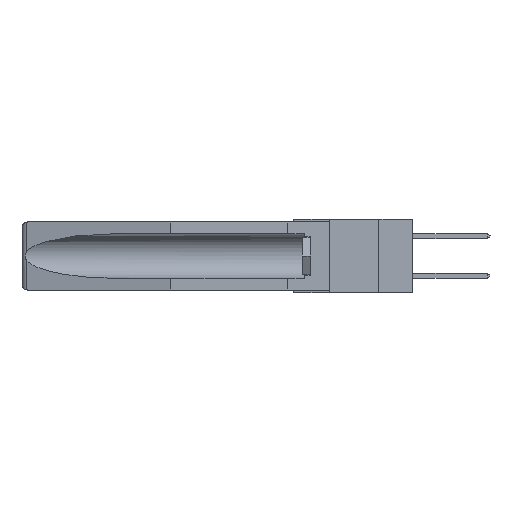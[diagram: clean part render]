
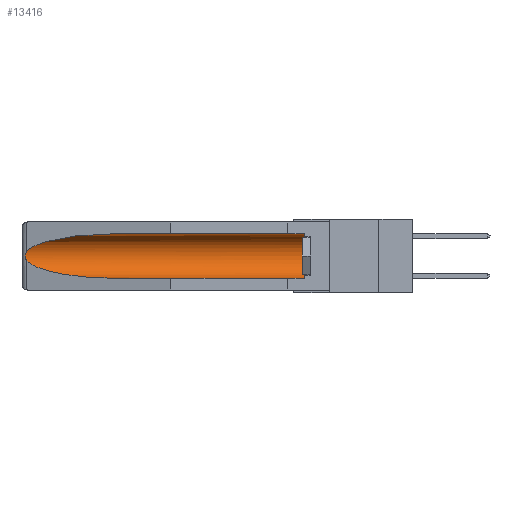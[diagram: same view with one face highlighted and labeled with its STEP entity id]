
A CAD part, left-side view. The second image highlights one B-rep face of the part: STEP entity #13416.
In plain terms, the highlighted cylindrical face has radius 2.857 mm (diameter 5.715 mm), a partial arc.
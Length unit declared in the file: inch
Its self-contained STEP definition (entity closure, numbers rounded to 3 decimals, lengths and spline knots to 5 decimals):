
#268 = CARTESIAN_POINT ( 'NONE',  ( 0.21114, 1.30732, -0.284 ) ) ;
#536 = DIRECTION ( 'NONE',  ( 0., 0., 1. ) ) ;
#1988 = LINE ( 'NONE', #3921, #26443 ) ;
#2520 = CARTESIAN_POINT ( 'NONE',  ( 0.2675, 1.53308, -0.17534 ) ) ;
#2658 = FACE_OUTER_BOUND ( 'NONE', #21291, .T. ) ;
#3213 = ORIENTED_EDGE ( 'NONE', *, *, #4659, .T. ) ;
#3408 = CYLINDRICAL_SURFACE ( 'NONE', #22263, 0.1125 ) ;
#3654 = EDGE_CURVE ( 'NONE', #27541, #6401, #23928, .T. ) ;
#3921 = CARTESIAN_POINT ( 'NONE',  ( 0.155, -0.30754, -0.059 ) ) ;
#4659 = EDGE_CURVE ( 'NONE', #10748, #25160, #1988, .T. ) ;
#5282 = CARTESIAN_POINT ( 'NONE',  ( 0.26537, 1.52718, -0.14972 ) ) ;
#6401 = VERTEX_POINT ( 'NONE', #11095 ) ;
#6407 = CARTESIAN_POINT ( 'NONE',  ( 0.155, 1.07973, -0.059 ) ) ;
#6480 = VECTOR ( 'NONE', #16291, 39.37008 ) ;
#7363 = CARTESIAN_POINT ( 'NONE',  ( 0.26597, 1.52961, -0.15275 ) ) ;
#7473 = CARTESIAN_POINT ( 'NONE',  ( 0.2673, 1.5327, -0.16383 ) ) ;
#7958 = CARTESIAN_POINT ( 'NONE',  ( 0.26537, 1.52718, -0.19328 ) ) ;
#8091 = ORIENTED_EDGE ( 'NONE', *, *, #16795, .T. ) ;
#9112 = CARTESIAN_POINT ( 'NONE',  ( 0.155, 0.126, -0.284 ) ) ;
#9590 = CIRCLE ( 'NONE', #29709, 0.1125 ) ;
#9718 = CARTESIAN_POINT ( 'NONE',  ( 0.26597, 1.5296, -0.19026 ) ) ;
#10748 = VERTEX_POINT ( 'NONE', #13776 ) ;
#11095 = CARTESIAN_POINT ( 'NONE',  ( 0.155, 1.07973, -0.284 ) ) ;
#11285 = EDGE_CURVE ( 'NONE', #25160, #21523, #18745, .T. ) ;
#11732 = CARTESIAN_POINT ( 'NONE',  ( 0.25451, 1.48313, -0.24835 ) ) ;
#12219 = CARTESIAN_POINT ( 'NONE',  ( 0.155, 1.07973, -0.059 ) ) ;
#12221 = CARTESIAN_POINT ( 'NONE',  ( 0.26654, 1.53092, -0.15636 ) ) ;
#13416 = ADVANCED_FACE ( 'NONE', ( #2658 ), #3408, .F. ) ;
#13776 = CARTESIAN_POINT ( 'NONE',  ( 0.155, 0.126, -0.059 ) ) ;
#13847 = CARTESIAN_POINT ( 'NONE',  ( 0.26537, 1.52718, -0.14972 ) ) ;
#15206 = ORIENTED_EDGE ( 'NONE', *, *, #3654, .F. ) ;
#16058 =( BOUNDED_CURVE ( )  B_SPLINE_CURVE ( 3, ( #28630, #11732, #268, #21120 ),
 .UNSPECIFIED., .F., .F. ) 
 B_SPLINE_CURVE_WITH_KNOTS ( ( 4, 4 ),
 ( 0.1948, 1.5708 ),
 .UNSPECIFIED. ) 
 CURVE ( )  GEOMETRIC_REPRESENTATION_ITEM ( )  RATIONAL_B_SPLINE_CURVE ( ( 1., 0.848, 0.848, 1. ) ) 
 REPRESENTATION_ITEM ( '' )  );
#16282 = CARTESIAN_POINT ( 'NONE',  ( 0.25451, 1.48313, -0.09465 ) ) ;
#16291 = DIRECTION ( 'NONE',  ( 0., 1., 0. ) ) ;
#16485 = ORIENTED_EDGE ( 'NONE', *, *, #28296, .T. ) ;
#16735 = CARTESIAN_POINT ( 'NONE',  ( 0.26537, 1.52718, -0.14972 ) ) ;
#16795 = EDGE_CURVE ( 'NONE', #21523, #22930, #18353, .T. ) ;
#17020 = CARTESIAN_POINT ( 'NONE',  ( 0.155, -0.30754, -0.1715 ) ) ;
#17056 = CARTESIAN_POINT ( 'NONE',  ( 0.26537, 1.52718, -0.19328 ) ) ;
#18353 = B_SPLINE_CURVE_WITH_KNOTS ( 'NONE', 3,
 ( #16735, #7363, #12221, #7473, #23977, #2520, #21411, #26237, #9718, #17056 ),
 .UNSPECIFIED., .F., .F.,
 ( 4, 2, 2, 2, 4 ),
 ( 0., 0.00029, 0.00058, 0.00087, 0.00117 ),
 .UNSPECIFIED. ) ;
#18745 =( BOUNDED_CURVE ( )  B_SPLINE_CURVE ( 3, ( #6407, #27965, #16282, #13847 ),
 .UNSPECIFIED., .F., .F. ) 
 B_SPLINE_CURVE_WITH_KNOTS ( ( 4, 4 ),
 ( 4.71239, 6.08839 ),
 .UNSPECIFIED. ) 
 CURVE ( )  GEOMETRIC_REPRESENTATION_ITEM ( )  RATIONAL_B_SPLINE_CURVE ( ( 1., 0.848, 0.848, 1. ) ) 
 REPRESENTATION_ITEM ( '' )  );
#18753 = ORIENTED_EDGE ( 'NONE', *, *, #30507, .T. ) ;
#19201 = DIRECTION ( 'NONE',  ( 0., 0., 1. ) ) ;
#21120 = CARTESIAN_POINT ( 'NONE',  ( 0.155, 1.07973, -0.284 ) ) ;
#21291 = EDGE_LOOP ( 'NONE', ( #23433, #8091, #16485, #15206, #18753, #3213 ) ) ;
#21388 = CARTESIAN_POINT ( 'NONE',  ( 0.155, 0.126, -0.1715 ) ) ;
#21411 = CARTESIAN_POINT ( 'NONE',  ( 0.2673, 1.53269, -0.17917 ) ) ;
#21523 = VERTEX_POINT ( 'NONE', #5282 ) ;
#22263 = AXIS2_PLACEMENT_3D ( 'NONE', #17020, #28895, #536 ) ;
#22930 = VERTEX_POINT ( 'NONE', #7958 ) ;
#23433 = ORIENTED_EDGE ( 'NONE', *, *, #11285, .T. ) ;
#23928 = LINE ( 'NONE', #30127, #6480 ) ;
#23977 = CARTESIAN_POINT ( 'NONE',  ( 0.2675, 1.53308, -0.16763 ) ) ;
#25160 = VERTEX_POINT ( 'NONE', #12219 ) ;
#25747 = DIRECTION ( 'NONE',  ( 0., 1., 0. ) ) ;
#26216 = DIRECTION ( 'NONE',  ( 0., -1., 0. ) ) ;
#26237 = CARTESIAN_POINT ( 'NONE',  ( 0.26655, 1.53094, -0.18657 ) ) ;
#26443 = VECTOR ( 'NONE', #25747, 39.37008 ) ;
#27541 = VERTEX_POINT ( 'NONE', #9112 ) ;
#27965 = CARTESIAN_POINT ( 'NONE',  ( 0.21114, 1.30732, -0.059 ) ) ;
#28296 = EDGE_CURVE ( 'NONE', #22930, #6401, #16058, .T. ) ;
#28630 = CARTESIAN_POINT ( 'NONE',  ( 0.26537, 1.52718, -0.19328 ) ) ;
#28895 = DIRECTION ( 'NONE',  ( 0., 1., 0. ) ) ;
#29709 = AXIS2_PLACEMENT_3D ( 'NONE', #21388, #26216, #19201 ) ;
#30127 = CARTESIAN_POINT ( 'NONE',  ( 0.155, -0.30754, -0.284 ) ) ;
#30507 = EDGE_CURVE ( 'NONE', #27541, #10748, #9590, .T. ) ;
